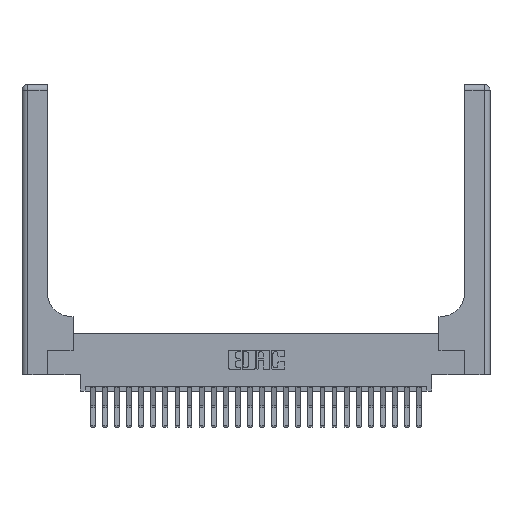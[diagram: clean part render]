
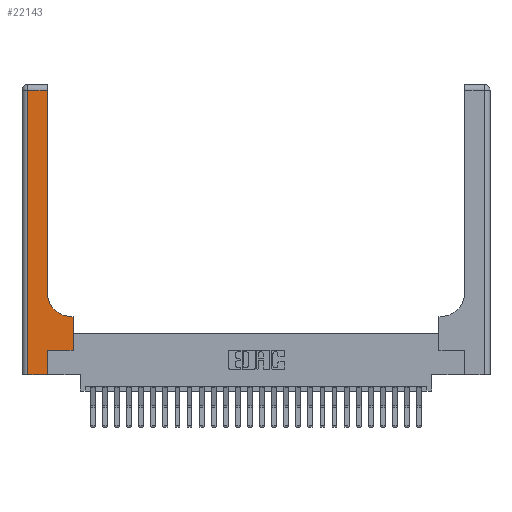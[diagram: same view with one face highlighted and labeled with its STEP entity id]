
A CAD part, top view. The second image highlights one B-rep face of the part: STEP entity #22143.
In plain terms, the highlighted planar face has unit normal (0, 0, 1).
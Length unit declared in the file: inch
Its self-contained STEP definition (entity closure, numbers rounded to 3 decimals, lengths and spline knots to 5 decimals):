
#234 = CARTESIAN_POINT ( 'NONE',  ( 0.26, 3., 0.37 ) ) ;
#708 = EDGE_CURVE ( 'NONE', #12555, #15310, #2540, .T. ) ;
#1164 = ORIENTED_EDGE ( 'NONE', *, *, #20621, .T. ) ;
#1367 = VECTOR ( 'NONE', #20939, 39.37008 ) ;
#1658 = CARTESIAN_POINT ( 'NONE',  ( 0., 3., 0.37 ) ) ;
#1994 = LINE ( 'NONE', #5136, #1367 ) ;
#2182 = EDGE_CURVE ( 'NONE', #19770, #4459, #3205, .T. ) ;
#2329 = LINE ( 'NONE', #8458, #17531 ) ;
#2540 = LINE ( 'NONE', #3634, #22954 ) ;
#2682 = VERTEX_POINT ( 'NONE', #21328 ) ;
#3205 = LINE ( 'NONE', #234, #3844 ) ;
#3634 = CARTESIAN_POINT ( 'NONE',  ( 0.26, 0.6, 0.37 ) ) ;
#3671 = ORIENTED_EDGE ( 'NONE', *, *, #3826, .T. ) ;
#3826 = EDGE_CURVE ( 'NONE', #4459, #18096, #15217, .T. ) ;
#3844 = VECTOR ( 'NONE', #14132, 39.37008 ) ;
#3975 = LINE ( 'NONE', #10664, #24316 ) ;
#4381 = CARTESIAN_POINT ( 'NONE',  ( 0.26, 2.94, 0.37 ) ) ;
#4459 = VERTEX_POINT ( 'NONE', #4381 ) ;
#5136 = CARTESIAN_POINT ( 'NONE',  ( 0.528, 0.25, 0.37 ) ) ;
#5158 = CARTESIAN_POINT ( 'NONE',  ( 0.26, 0.85, 0.37 ) ) ;
#5306 = CARTESIAN_POINT ( 'NONE',  ( 0.51, 0.85, 0.37 ) ) ;
#5651 = DIRECTION ( 'NONE',  ( 0., 0., -1. ) ) ;
#7326 = DIRECTION ( 'NONE',  ( 1., 0., 0. ) ) ;
#8458 = CARTESIAN_POINT ( 'NONE',  ( 0.06, 3., 0.37 ) ) ;
#8749 = DIRECTION ( 'NONE',  ( 1., 0., 0. ) ) ;
#8977 = CARTESIAN_POINT ( 'NONE',  ( 0.265, 0., 0.37 ) ) ;
#9292 = EDGE_LOOP ( 'NONE', ( #22210, #3671, #21920, #12049, #22515, #1164, #11747, #17643, #15164 ) ) ;
#9755 = LINE ( 'NONE', #22324, #14388 ) ;
#9975 = VECTOR ( 'NONE', #14525, 39.37008 ) ;
#10132 = CARTESIAN_POINT ( 'NONE',  ( 0.265, 0.25, 0.37 ) ) ;
#10478 = CARTESIAN_POINT ( 'NONE',  ( 0., 2.94, 0.37 ) ) ;
#10664 = CARTESIAN_POINT ( 'NONE',  ( 0.265, 0.25, 0.37 ) ) ;
#11747 = ORIENTED_EDGE ( 'NONE', *, *, #15175, .T. ) ;
#12049 = ORIENTED_EDGE ( 'NONE', *, *, #15514, .T. ) ;
#12480 = DIRECTION ( 'NONE',  ( 1., 0., 0. ) ) ;
#12555 = VERTEX_POINT ( 'NONE', #22975 ) ;
#13593 = DIRECTION ( 'NONE',  ( -1., 0., 0. ) ) ;
#13822 = FACE_OUTER_BOUND ( 'NONE', #9292, .T. ) ;
#13907 = CARTESIAN_POINT ( 'NONE',  ( 0.51, 0.6, 0.37 ) ) ;
#14132 = DIRECTION ( 'NONE',  ( 0., 1., 0. ) ) ;
#14388 = VECTOR ( 'NONE', #12480, 39.37008 ) ;
#14525 = DIRECTION ( 'NONE',  ( -1., 0., 0. ) ) ;
#14923 = EDGE_CURVE ( 'NONE', #18096, #25021, #2329, .T. ) ;
#15164 = ORIENTED_EDGE ( 'NONE', *, *, #22032, .T. ) ;
#15175 = EDGE_CURVE ( 'NONE', #17487, #12555, #1994, .T. ) ;
#15217 = LINE ( 'NONE', #10478, #9975 ) ;
#15310 = VERTEX_POINT ( 'NONE', #13907 ) ;
#15514 = EDGE_CURVE ( 'NONE', #25021, #2682, #9755, .T. ) ;
#17219 = AXIS2_PLACEMENT_3D ( 'NONE', #1658, #5651, #19492 ) ;
#17275 = CARTESIAN_POINT ( 'NONE',  ( 0.06, 2.94, 0.37 ) ) ;
#17487 = VERTEX_POINT ( 'NONE', #25088 ) ;
#17531 = VECTOR ( 'NONE', #22262, 39.37008 ) ;
#17643 = ORIENTED_EDGE ( 'NONE', *, *, #708, .T. ) ;
#18096 = VERTEX_POINT ( 'NONE', #17275 ) ;
#18966 = VECTOR ( 'NONE', #22767, 39.37008 ) ;
#19151 = DIRECTION ( 'NONE',  ( 0., 0., -1. ) ) ;
#19468 = VERTEX_POINT ( 'NONE', #10132 ) ;
#19492 = DIRECTION ( 'NONE',  ( -1., 0., 0. ) ) ;
#19770 = VERTEX_POINT ( 'NONE', #5158 ) ;
#20621 = EDGE_CURVE ( 'NONE', #19468, #17487, #3975, .T. ) ;
#20939 = DIRECTION ( 'NONE',  ( 0., 1., 0. ) ) ;
#21328 = CARTESIAN_POINT ( 'NONE',  ( 0.265, 0., 0.37 ) ) ;
#21526 = CIRCLE ( 'NONE', #25582, 0.25 ) ;
#21920 = ORIENTED_EDGE ( 'NONE', *, *, #14923, .T. ) ;
#22032 = EDGE_CURVE ( 'NONE', #15310, #19770, #21526, .T. ) ;
#22143 = ADVANCED_FACE ( 'NONE', ( #13822 ), #25293, .F. ) ;
#22210 = ORIENTED_EDGE ( 'NONE', *, *, #2182, .T. ) ;
#22262 = DIRECTION ( 'NONE',  ( 0., -1., 0. ) ) ;
#22295 = CARTESIAN_POINT ( 'NONE',  ( 0.06, 0., 0.37 ) ) ;
#22324 = CARTESIAN_POINT ( 'NONE',  ( 0., 0., 0.37 ) ) ;
#22515 = ORIENTED_EDGE ( 'NONE', *, *, #23914, .T. ) ;
#22767 = DIRECTION ( 'NONE',  ( 0., 1., 0. ) ) ;
#22954 = VECTOR ( 'NONE', #13593, 39.37008 ) ;
#22975 = CARTESIAN_POINT ( 'NONE',  ( 0.528, 0.6, 0.37 ) ) ;
#23584 = LINE ( 'NONE', #8977, #18966 ) ;
#23914 = EDGE_CURVE ( 'NONE', #2682, #19468, #23584, .T. ) ;
#24316 = VECTOR ( 'NONE', #8749, 39.37008 ) ;
#25021 = VERTEX_POINT ( 'NONE', #22295 ) ;
#25088 = CARTESIAN_POINT ( 'NONE',  ( 0.528, 0.25, 0.37 ) ) ;
#25293 = PLANE ( 'NONE',  #17219 ) ;
#25582 = AXIS2_PLACEMENT_3D ( 'NONE', #5306, #19151, #7326 ) ;
